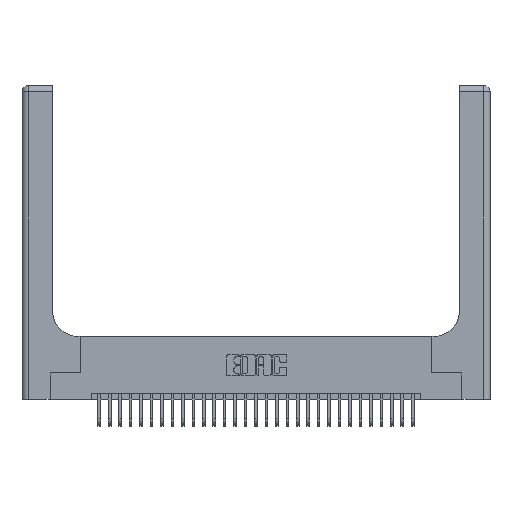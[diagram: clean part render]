
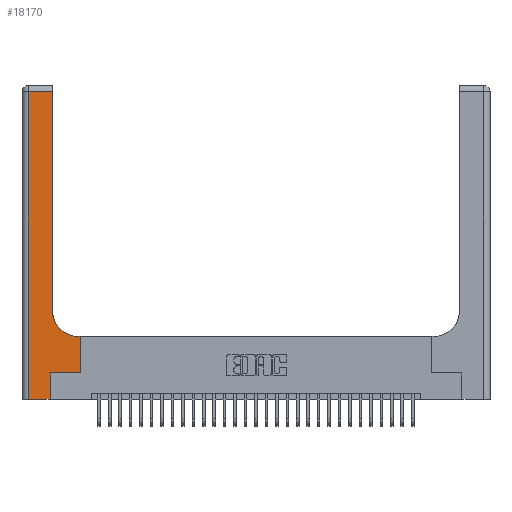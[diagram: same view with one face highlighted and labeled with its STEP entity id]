
A CAD part, top view. The second image highlights one B-rep face of the part: STEP entity #18170.
In plain terms, the highlighted planar face has unit normal (0, 0, 1).
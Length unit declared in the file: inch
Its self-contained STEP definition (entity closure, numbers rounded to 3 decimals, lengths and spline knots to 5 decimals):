
#232 = VECTOR ( 'NONE', #5124, 39.37008 ) ;
#321 = EDGE_CURVE ( 'NONE', #1489, #4058, #14093, .T. ) ;
#422 = ORIENTED_EDGE ( 'NONE', *, *, #13810, .T. ) ;
#467 = AXIS2_PLACEMENT_3D ( 'NONE', #9746, #25894, #12093 ) ;
#679 = CARTESIAN_POINT ( 'NONE',  ( 0., 3., 0.37 ) ) ;
#1489 = VERTEX_POINT ( 'NONE', #8274 ) ;
#1556 = VECTOR ( 'NONE', #12868, 39.37008 ) ;
#2853 = CARTESIAN_POINT ( 'NONE',  ( 0.2915, 0.6, 0.37 ) ) ;
#2893 = EDGE_CURVE ( 'NONE', #17029, #10160, #20891, .T. ) ;
#3042 = DIRECTION ( 'NONE',  ( -1., 0., 0. ) ) ;
#3276 = EDGE_LOOP ( 'NONE', ( #24818, #5223, #7659, #16340, #10928, #10988, #7070, #422, #29494 ) ) ;
#3545 = DIRECTION ( 'NONE',  ( 0., 1., 0. ) ) ;
#4058 = VERTEX_POINT ( 'NONE', #4951 ) ;
#4653 = DIRECTION ( 'NONE',  ( 1., 0., 0. ) ) ;
#4951 = CARTESIAN_POINT ( 'NONE',  ( 0.5585, 0.25, 0.37 ) ) ;
#5053 = VERTEX_POINT ( 'NONE', #15461 ) ;
#5124 = DIRECTION ( 'NONE',  ( -1., 0., 0. ) ) ;
#5223 = ORIENTED_EDGE ( 'NONE', *, *, #21246, .T. ) ;
#6157 = DIRECTION ( 'NONE',  ( 0., -1., 0. ) ) ;
#6305 = EDGE_CURVE ( 'NONE', #10160, #1489, #10155, .T. ) ;
#7070 = ORIENTED_EDGE ( 'NONE', *, *, #12084, .T. ) ;
#7659 = ORIENTED_EDGE ( 'NONE', *, *, #11290, .T. ) ;
#7822 = CARTESIAN_POINT ( 'NONE',  ( 0.06, 0., 0.37 ) ) ;
#7856 = VECTOR ( 'NONE', #8627, 39.37008 ) ;
#8274 = CARTESIAN_POINT ( 'NONE',  ( 0.269, 0.25, 0.37 ) ) ;
#8627 = DIRECTION ( 'NONE',  ( 1., 0., 0. ) ) ;
#8862 = CARTESIAN_POINT ( 'NONE',  ( 0.5415, 0.6, 0.37 ) ) ;
#8906 = CARTESIAN_POINT ( 'NONE',  ( 0.269, 0., 0.37 ) ) ;
#9112 = VERTEX_POINT ( 'NONE', #18868 ) ;
#9193 = FACE_OUTER_BOUND ( 'NONE', #3276, .T. ) ;
#9295 = CARTESIAN_POINT ( 'NONE',  ( 0.06, 3., 0.37 ) ) ;
#9746 = CARTESIAN_POINT ( 'NONE',  ( 0.5415, 0.85, 0.37 ) ) ;
#10155 = LINE ( 'NONE', #24427, #14168 ) ;
#10160 = VERTEX_POINT ( 'NONE', #8906 ) ;
#10928 = ORIENTED_EDGE ( 'NONE', *, *, #6305, .T. ) ;
#10988 = ORIENTED_EDGE ( 'NONE', *, *, #321, .T. ) ;
#11290 = EDGE_CURVE ( 'NONE', #29493, #17029, #28472, .T. ) ;
#11638 = LINE ( 'NONE', #13312, #29249 ) ;
#11663 = CARTESIAN_POINT ( 'NONE',  ( 0., 0., 0.37 ) ) ;
#11673 = VERTEX_POINT ( 'NONE', #8862 ) ;
#12084 = EDGE_CURVE ( 'NONE', #4058, #5053, #22379, .T. ) ;
#12093 = DIRECTION ( 'NONE',  ( 1., 0., 0. ) ) ;
#12788 = LINE ( 'NONE', #2853, #232 ) ;
#12868 = DIRECTION ( 'NONE',  ( 0., 1., 0. ) ) ;
#13312 = CARTESIAN_POINT ( 'NONE',  ( 0.2915, 3., 0.37 ) ) ;
#13810 = EDGE_CURVE ( 'NONE', #5053, #11673, #12788, .T. ) ;
#14066 = CARTESIAN_POINT ( 'NONE',  ( 0.2915, 2.94, 0.37 ) ) ;
#14093 = LINE ( 'NONE', #29271, #7856 ) ;
#14133 = VECTOR ( 'NONE', #6157, 39.37008 ) ;
#14168 = VECTOR ( 'NONE', #3545, 39.37008 ) ;
#14757 = VECTOR ( 'NONE', #4653, 39.37008 ) ;
#14775 = PLANE ( 'NONE',  #23299 ) ;
#15461 = CARTESIAN_POINT ( 'NONE',  ( 0.5585, 0.6, 0.37 ) ) ;
#16340 = ORIENTED_EDGE ( 'NONE', *, *, #2893, .T. ) ;
#17029 = VERTEX_POINT ( 'NONE', #7822 ) ;
#17090 = DIRECTION ( 'NONE',  ( 0., 0., -1. ) ) ;
#17700 = LINE ( 'NONE', #20330, #19862 ) ;
#17960 = DIRECTION ( 'NONE',  ( 0., 1., 0. ) ) ;
#18170 = ADVANCED_FACE ( 'NONE', ( #9193 ), #14775, .F. ) ;
#18868 = CARTESIAN_POINT ( 'NONE',  ( 0.2915, 0.85, 0.37 ) ) ;
#19862 = VECTOR ( 'NONE', #27211, 39.37008 ) ;
#20282 = EDGE_CURVE ( 'NONE', #11673, #9112, #29173, .T. ) ;
#20330 = CARTESIAN_POINT ( 'NONE',  ( 0., 2.94, 0.37 ) ) ;
#20891 = LINE ( 'NONE', #11663, #14757 ) ;
#21246 = EDGE_CURVE ( 'NONE', #21361, #29493, #17700, .T. ) ;
#21361 = VERTEX_POINT ( 'NONE', #14066 ) ;
#22379 = LINE ( 'NONE', #26525, #1556 ) ;
#23299 = AXIS2_PLACEMENT_3D ( 'NONE', #679, #17090, #3042 ) ;
#24427 = CARTESIAN_POINT ( 'NONE',  ( 0.269, 0., 0.37 ) ) ;
#24818 = ORIENTED_EDGE ( 'NONE', *, *, #27995, .T. ) ;
#24936 = CARTESIAN_POINT ( 'NONE',  ( 0.06, 2.94, 0.37 ) ) ;
#25894 = DIRECTION ( 'NONE',  ( 0., 0., -1. ) ) ;
#26525 = CARTESIAN_POINT ( 'NONE',  ( 0.5585, 0.25, 0.37 ) ) ;
#27211 = DIRECTION ( 'NONE',  ( -1., 0., 0. ) ) ;
#27995 = EDGE_CURVE ( 'NONE', #9112, #21361, #11638, .T. ) ;
#28472 = LINE ( 'NONE', #9295, #14133 ) ;
#29173 = CIRCLE ( 'NONE', #467, 0.25 ) ;
#29249 = VECTOR ( 'NONE', #17960, 39.37008 ) ;
#29271 = CARTESIAN_POINT ( 'NONE',  ( 0.269, 0.25, 0.37 ) ) ;
#29493 = VERTEX_POINT ( 'NONE', #24936 ) ;
#29494 = ORIENTED_EDGE ( 'NONE', *, *, #20282, .T. ) ;
